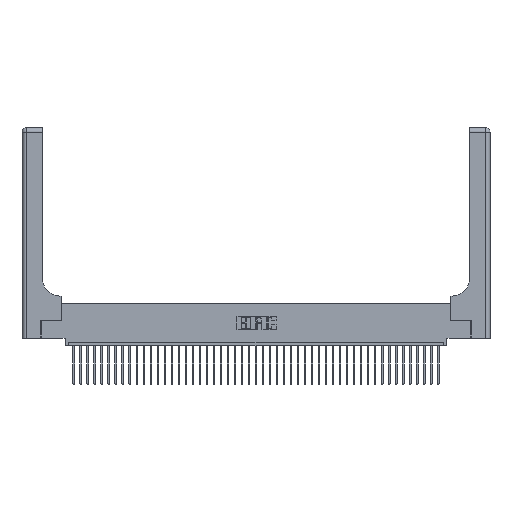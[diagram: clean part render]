
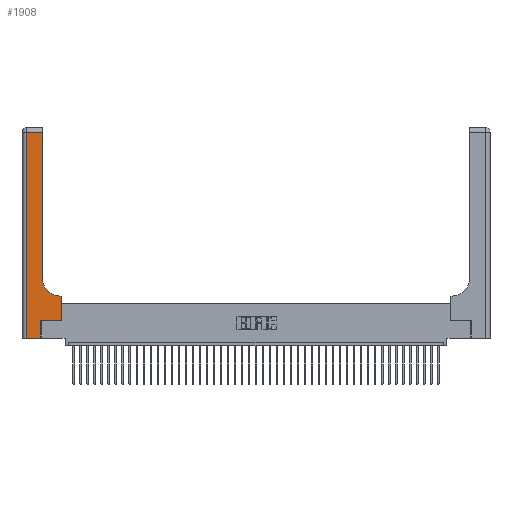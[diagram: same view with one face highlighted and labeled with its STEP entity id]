
A CAD part, top view. The second image highlights one B-rep face of the part: STEP entity #1908.
In plain terms, the highlighted planar face has unit normal (0, 0, 1).
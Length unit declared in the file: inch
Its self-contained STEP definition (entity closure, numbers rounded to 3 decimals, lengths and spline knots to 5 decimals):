
#432 = VECTOR ( 'NONE', #39995, 39.37008 ) ;
#578 = CARTESIAN_POINT ( 'NONE',  ( 0., 0., 0.37 ) ) ;
#693 = EDGE_CURVE ( 'NONE', #10590, #26542, #1743, .T. ) ;
#730 = ORIENTED_EDGE ( 'NONE', *, *, #693, .T. ) ;
#916 = DIRECTION ( 'NONE',  ( 1., 0., 0. ) ) ;
#1070 = AXIS2_PLACEMENT_3D ( 'NONE', #43027, #35919, #12627 ) ;
#1586 = CARTESIAN_POINT ( 'NONE',  ( 0.06, 3., 0.37 ) ) ;
#1743 = LINE ( 'NONE', #12790, #41931 ) ;
#1770 = DIRECTION ( 'NONE',  ( -1., 0., 0. ) ) ;
#1908 = ADVANCED_FACE ( 'NONE', ( #37600 ), #32543, .F. ) ;
#1951 = LINE ( 'NONE', #20438, #9398 ) ;
#2776 = EDGE_CURVE ( 'NONE', #19361, #4518, #18539, .T. ) ;
#3265 = VERTEX_POINT ( 'NONE', #27027 ) ;
#3526 = VECTOR ( 'NONE', #30595, 39.37008 ) ;
#4275 = CARTESIAN_POINT ( 'NONE',  ( 0., 2.94, 0.37 ) ) ;
#4518 = VERTEX_POINT ( 'NONE', #26886 ) ;
#5933 = DIRECTION ( 'NONE',  ( 0., 1., 0. ) ) ;
#6865 = VECTOR ( 'NONE', #38020, 39.37008 ) ;
#6903 = ORIENTED_EDGE ( 'NONE', *, *, #18169, .T. ) ;
#7298 = CARTESIAN_POINT ( 'NONE',  ( 0.06, 2.94, 0.37 ) ) ;
#7711 = DIRECTION ( 'NONE',  ( 0., 0., -1. ) ) ;
#7734 = EDGE_CURVE ( 'NONE', #41397, #38150, #23320, .T. ) ;
#7878 = EDGE_CURVE ( 'NONE', #38150, #34310, #15901, .T. ) ;
#9398 = VECTOR ( 'NONE', #24010, 39.37008 ) ;
#10590 = VERTEX_POINT ( 'NONE', #12406 ) ;
#10593 = LINE ( 'NONE', #4275, #15883 ) ;
#11736 = CARTESIAN_POINT ( 'NONE',  ( 0.5585, 0.25, 0.37 ) ) ;
#12406 = CARTESIAN_POINT ( 'NONE',  ( 0.269, 0.25, 0.37 ) ) ;
#12627 = DIRECTION ( 'NONE',  ( -1., 0., 0. ) ) ;
#12790 = CARTESIAN_POINT ( 'NONE',  ( 0.269, 0.25, 0.37 ) ) ;
#13051 = CARTESIAN_POINT ( 'NONE',  ( 0.269, 0., 0.37 ) ) ;
#13291 = CARTESIAN_POINT ( 'NONE',  ( 0.2915, 2.94, 0.37 ) ) ;
#13541 = EDGE_CURVE ( 'NONE', #3265, #41397, #1951, .T. ) ;
#15675 = VECTOR ( 'NONE', #5933, 39.37008 ) ;
#15883 = VECTOR ( 'NONE', #1770, 39.37008 ) ;
#15901 = LINE ( 'NONE', #31708, #6865 ) ;
#18169 = EDGE_CURVE ( 'NONE', #34310, #19361, #10593, .T. ) ;
#18539 = LINE ( 'NONE', #1586, #35904 ) ;
#19017 = VERTEX_POINT ( 'NONE', #13051 ) ;
#19075 = EDGE_CURVE ( 'NONE', #26542, #3265, #29543, .T. ) ;
#19361 = VERTEX_POINT ( 'NONE', #7298 ) ;
#19926 = CARTESIAN_POINT ( 'NONE',  ( 0.5415, 0.6, 0.37 ) ) ;
#20438 = CARTESIAN_POINT ( 'NONE',  ( 0.2915, 0.6, 0.37 ) ) ;
#20701 = ORIENTED_EDGE ( 'NONE', *, *, #28405, .T. ) ;
#20746 = EDGE_CURVE ( 'NONE', #4518, #19017, #37347, .T. ) ;
#23320 = CIRCLE ( 'NONE', #28389, 0.25 ) ;
#24010 = DIRECTION ( 'NONE',  ( -1., 0., 0. ) ) ;
#26263 = LINE ( 'NONE', #42994, #15675 ) ;
#26542 = VERTEX_POINT ( 'NONE', #11736 ) ;
#26886 = CARTESIAN_POINT ( 'NONE',  ( 0.06, 0., 0.37 ) ) ;
#27027 = CARTESIAN_POINT ( 'NONE',  ( 0.5585, 0.6, 0.37 ) ) ;
#28389 = AXIS2_PLACEMENT_3D ( 'NONE', #37625, #7711, #916 ) ;
#28405 = EDGE_CURVE ( 'NONE', #19017, #10590, #26263, .T. ) ;
#29543 = LINE ( 'NONE', #42947, #432 ) ;
#30208 = DIRECTION ( 'NONE',  ( 1., 0., 0. ) ) ;
#30595 = DIRECTION ( 'NONE',  ( 1., 0., 0. ) ) ;
#30720 = ORIENTED_EDGE ( 'NONE', *, *, #7734, .T. ) ;
#31623 = ORIENTED_EDGE ( 'NONE', *, *, #20746, .T. ) ;
#31666 = EDGE_LOOP ( 'NONE', ( #41470, #6903, #33523, #31623, #20701, #730, #37526, #37483, #30720 ) ) ;
#31708 = CARTESIAN_POINT ( 'NONE',  ( 0.2915, 3., 0.37 ) ) ;
#32543 = PLANE ( 'NONE',  #1070 ) ;
#33523 = ORIENTED_EDGE ( 'NONE', *, *, #2776, .T. ) ;
#34310 = VERTEX_POINT ( 'NONE', #13291 ) ;
#35904 = VECTOR ( 'NONE', #38652, 39.37008 ) ;
#35919 = DIRECTION ( 'NONE',  ( 0., 0., -1. ) ) ;
#37347 = LINE ( 'NONE', #578, #3526 ) ;
#37483 = ORIENTED_EDGE ( 'NONE', *, *, #13541, .T. ) ;
#37526 = ORIENTED_EDGE ( 'NONE', *, *, #19075, .T. ) ;
#37600 = FACE_OUTER_BOUND ( 'NONE', #31666, .T. ) ;
#37625 = CARTESIAN_POINT ( 'NONE',  ( 0.5415, 0.85, 0.37 ) ) ;
#38020 = DIRECTION ( 'NONE',  ( 0., 1., 0. ) ) ;
#38150 = VERTEX_POINT ( 'NONE', #42762 ) ;
#38652 = DIRECTION ( 'NONE',  ( 0., -1., 0. ) ) ;
#39995 = DIRECTION ( 'NONE',  ( 0., 1., 0. ) ) ;
#41397 = VERTEX_POINT ( 'NONE', #19926 ) ;
#41470 = ORIENTED_EDGE ( 'NONE', *, *, #7878, .T. ) ;
#41931 = VECTOR ( 'NONE', #30208, 39.37008 ) ;
#42762 = CARTESIAN_POINT ( 'NONE',  ( 0.2915, 0.85, 0.37 ) ) ;
#42947 = CARTESIAN_POINT ( 'NONE',  ( 0.5585, 0.25, 0.37 ) ) ;
#42994 = CARTESIAN_POINT ( 'NONE',  ( 0.269, 0., 0.37 ) ) ;
#43027 = CARTESIAN_POINT ( 'NONE',  ( 0., 3., 0.37 ) ) ;
